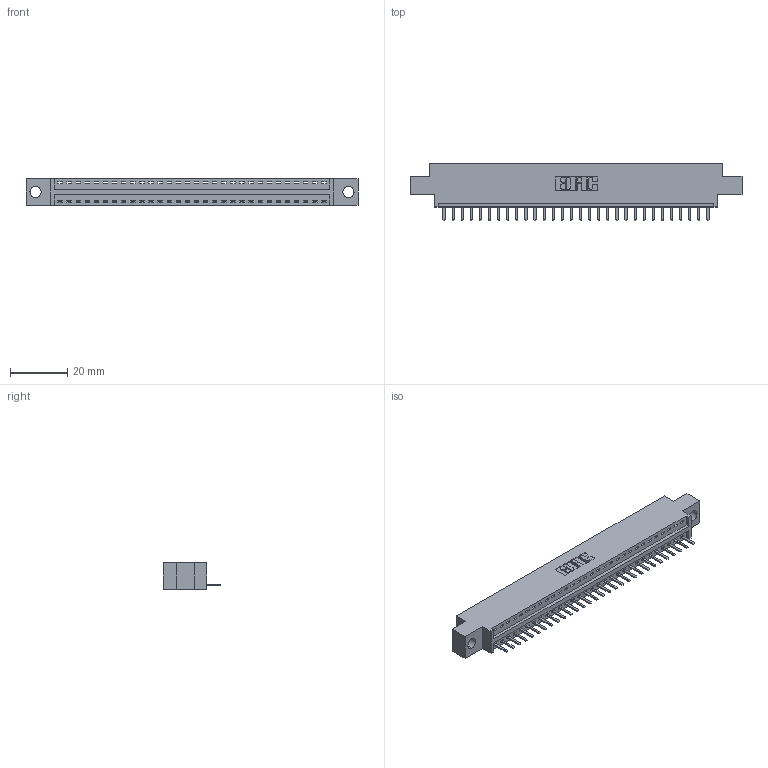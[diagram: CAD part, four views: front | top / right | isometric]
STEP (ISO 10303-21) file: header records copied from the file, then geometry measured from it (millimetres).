
FILE_DESCRIPTION (( 'STEP AP203' ), '1' );
FILE_NAME ('346-030-520-604.STEP', '2018-08-22T04:19:01', ( '' ), ( '' ), 'SwSTEP 2.0', 'SolidWorks 2016', '' );
FILE_SCHEMA (( 'CONFIG_CONTROL_DESIGN' ));
Length unit declared in the file: inch
Products named in the file (3): 346 Part_0.170 Offset - 0.156 Dia-TH; 345-292-001_345-293-120; 346-030-520-604
Assembly tree (31 placements, depth 2):
  346-030-520-604
    346 Part_0.170 Offset - 0.156 Dia-TH
    345-292-001_345-293-120  x30
Bounding box: 115.82 x 20.02 x 9.4 mm (x, y, z)
Volume: 10675.5 mm3; surface area: 12890.7 mm2
Topology: 31 solids, 31 shells, 1986 faces, 5861 edges, 3826 vertices
Faces by surface type: plane 1340, cylinder 646
Entity records: 20483 total; most frequent: CARTESIAN_POINT 3534, ORIENTED_EDGE 3486, DIRECTION 3119, EDGE_CURVE 1743, VECTOR 1487, LINE 1487, VERTEX_POINT 1158, AXIS2_PLACEMENT_3D 816
